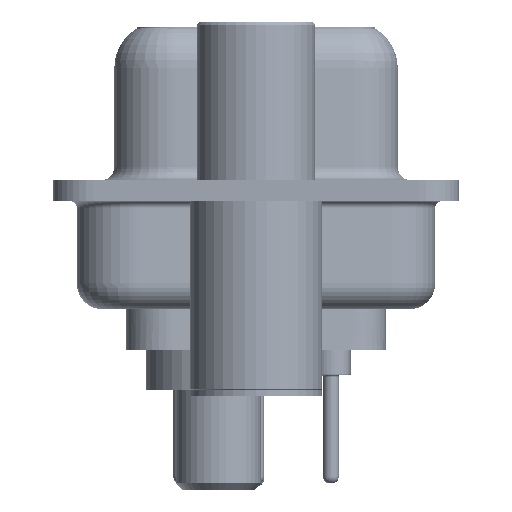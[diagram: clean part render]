
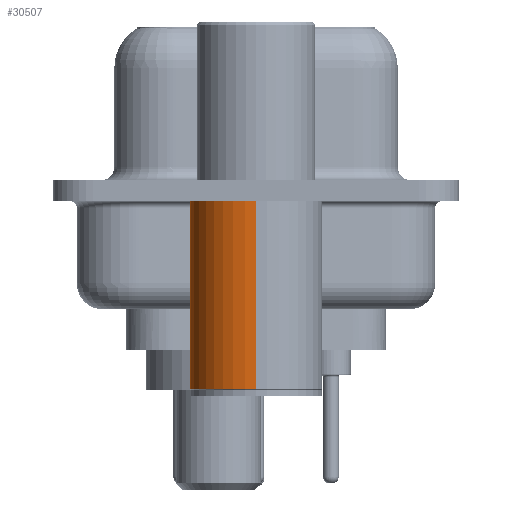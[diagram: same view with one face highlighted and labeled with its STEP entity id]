
A CAD part, left-side view. The second image highlights one B-rep face of the part: STEP entity #30507.
In plain terms, the highlighted cylindrical face has radius 2.5 mm (diameter 5 mm), a partial arc.
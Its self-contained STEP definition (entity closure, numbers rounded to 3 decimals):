
#591 = DIRECTION ( 'NONE',  ( 1., 0., 0. ) ) ;
#883 = DIRECTION ( 'NONE',  ( 0., 0., 1. ) ) ;
#1428 = CYLINDRICAL_SURFACE ( 'NONE', #8701, 2.5 ) ;
#1748 = DIRECTION ( 'NONE',  ( 1., 0., 0. ) ) ;
#2219 = VERTEX_POINT ( 'NONE', #23988 ) ;
#3478 = LINE ( 'NONE', #8815, #33064 ) ;
#3766 = VERTEX_POINT ( 'NONE', #7684 ) ;
#4425 = DIRECTION ( 'NONE',  ( 1., 0., 0. ) ) ;
#5577 = VECTOR ( 'NONE', #5972, 1000. ) ;
#5786 = CARTESIAN_POINT ( 'NONE',  ( 2.5, 0., -7.525 ) ) ;
#5972 = DIRECTION ( 'NONE',  ( 0., 0., 1. ) ) ;
#6109 = ORIENTED_EDGE ( 'NONE', *, *, #29954, .T. ) ;
#6132 = CARTESIAN_POINT ( 'NONE',  ( 0., 0., -7.525 ) ) ;
#7684 = CARTESIAN_POINT ( 'NONE',  ( -2.5, 0., -0.4 ) ) ;
#7689 = LINE ( 'NONE', #24874, #5577 ) ;
#7788 = EDGE_LOOP ( 'NONE', ( #6109, #9761, #12910, #12048 ) ) ;
#8701 = AXIS2_PLACEMENT_3D ( 'NONE', #20819, #23803, #4425 ) ;
#8815 = CARTESIAN_POINT ( 'NONE',  ( -2.5, 0., 0.581 ) ) ;
#9761 = ORIENTED_EDGE ( 'NONE', *, *, #32528, .T. ) ;
#10569 = VERTEX_POINT ( 'NONE', #15502 ) ;
#12048 = ORIENTED_EDGE ( 'NONE', *, *, #34871, .F. ) ;
#12910 = ORIENTED_EDGE ( 'NONE', *, *, #16829, .F. ) ;
#13366 = CIRCLE ( 'NONE', #35496, 2.5 ) ;
#15426 = CARTESIAN_POINT ( 'NONE',  ( 0., 0., -0.4 ) ) ;
#15502 = CARTESIAN_POINT ( 'NONE',  ( -2.5, 0., -7.525 ) ) ;
#15593 = AXIS2_PLACEMENT_3D ( 'NONE', #6132, #25151, #591 ) ;
#16829 = EDGE_CURVE ( 'NONE', #2219, #3766, #13366, .T. ) ;
#20819 = CARTESIAN_POINT ( 'NONE',  ( 0., 0., 0.581 ) ) ;
#22715 = DIRECTION ( 'NONE',  ( 0., 0., 1. ) ) ;
#23803 = DIRECTION ( 'NONE',  ( 0., 0., 1. ) ) ;
#23988 = CARTESIAN_POINT ( 'NONE',  ( 2.5, 0., -0.4 ) ) ;
#24874 = CARTESIAN_POINT ( 'NONE',  ( 2.5, 0., 0.581 ) ) ;
#25151 = DIRECTION ( 'NONE',  ( 0., 0., 1. ) ) ;
#27128 = CIRCLE ( 'NONE', #15593, 2.5 ) ;
#28784 = VERTEX_POINT ( 'NONE', #5786 ) ;
#29954 = EDGE_CURVE ( 'NONE', #28784, #10569, #27128, .T. ) ;
#30507 = ADVANCED_FACE ( 'NONE', ( #31463 ), #1428, .T. ) ;
#31463 = FACE_OUTER_BOUND ( 'NONE', #7788, .T. ) ;
#32528 = EDGE_CURVE ( 'NONE', #10569, #3766, #3478, .T. ) ;
#33064 = VECTOR ( 'NONE', #883, 1000. ) ;
#34871 = EDGE_CURVE ( 'NONE', #28784, #2219, #7689, .T. ) ;
#35496 = AXIS2_PLACEMENT_3D ( 'NONE', #15426, #22715, #1748 ) ;
